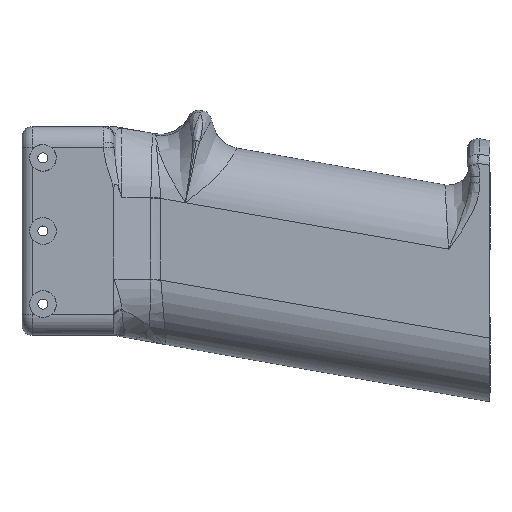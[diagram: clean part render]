
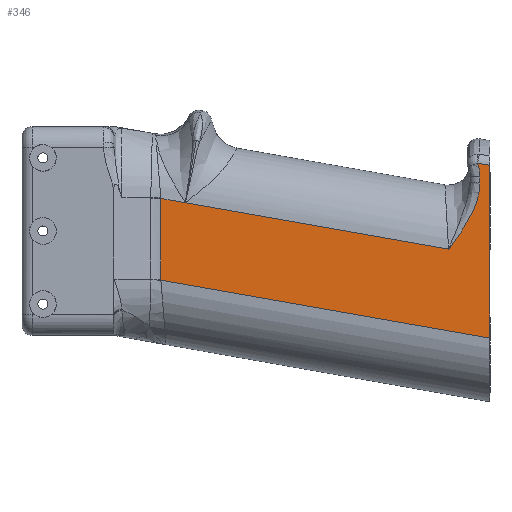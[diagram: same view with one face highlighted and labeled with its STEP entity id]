
A CAD part, left-side view. The second image highlights one B-rep face of the part: STEP entity #346.
In plain terms, the highlighted planar face has unit normal (-1, 0, 0).
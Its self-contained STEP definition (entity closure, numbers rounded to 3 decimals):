
#270 = CARTESIAN_POINT ( 'NONE',  ( 2.5, -96.204, 16.387 ) ) ;
#346 = ADVANCED_FACE ( 'NONE', ( #710 ), #13445, .F. ) ;
#477 = LINE ( 'NONE', #270, #973 ) ;
#658 = LINE ( 'NONE', #7215, #9537 ) ;
#710 = FACE_OUTER_BOUND ( 'NONE', #6651, .T. ) ;
#736 = CARTESIAN_POINT ( 'NONE',  ( 2.5, -97.508, 10.008 ) ) ;
#790 = CARTESIAN_POINT ( 'NONE',  ( 2.5, -91.197, -2.863 ) ) ;
#973 = VECTOR ( 'NONE', #2447, 1000. ) ;
#1314 = VECTOR ( 'NONE', #1765, 1000. ) ;
#1408 = VERTEX_POINT ( 'NONE', #7202 ) ;
#1598 = CARTESIAN_POINT ( 'NONE',  ( 2.5, -97.358, 15.166 ) ) ;
#1765 = DIRECTION ( 'NONE',  ( 0., -0.985, -0.174 ) ) ;
#1837 = CARTESIAN_POINT ( 'NONE',  ( 2.5, -97.089, 7.821 ) ) ;
#1891 = CARTESIAN_POINT ( 'NONE',  ( 2.5, -90.525, -3.757 ) ) ;
#1935 = AXIS2_PLACEMENT_3D ( 'NONE', #3222, #5436, #13278 ) ;
#2315 = ORIENTED_EDGE ( 'NONE', *, *, #8840, .T. ) ;
#2447 = DIRECTION ( 'NONE',  ( 0., 0.985, 0.174 ) ) ;
#2693 = CARTESIAN_POINT ( 'NONE',  ( 2.5, -97.045, 16.238 ) ) ;
#2938 = CARTESIAN_POINT ( 'NONE',  ( 2.5, -96.634, 6.394 ) ) ;
#2992 = CARTESIAN_POINT ( 'NONE',  ( 2.5, -90.076, -4.351 ) ) ;
#3032 = VERTEX_POINT ( 'NONE', #5212 ) ;
#3222 = CARTESIAN_POINT ( 'NONE',  ( 2.5, 0., 0. ) ) ;
#3355 = B_SPLINE_CURVE_WITH_KNOTS ( 'NONE', 3,
 ( #2693, #9394, #1598, #10521, #3806, #11645 ),
 .UNSPECIFIED., .F., .F.,
 ( 4, 2, 4 ),
 ( 0.001, 0.003, 0.004 ),
 .UNSPECIFIED. ) ;
#3390 = CARTESIAN_POINT ( 'NONE',  ( 2.5, -100., 15.717 ) ) ;
#3616 = CARTESIAN_POINT ( 'NONE',  ( 2.5, -97.576, 12.93 ) ) ;
#3806 = CARTESIAN_POINT ( 'NONE',  ( 2.5, -97.576, 13.493 ) ) ;
#4048 = CARTESIAN_POINT ( 'NONE',  ( 2.5, -96.231, 5.351 ) ) ;
#4054 = ORIENTED_EDGE ( 'NONE', *, *, #8875, .T. ) ;
#4249 = LINE ( 'NONE', #7754, #8971 ) ;
#4265 = VERTEX_POINT ( 'NONE', #5051 ) ;
#4573 = LINE ( 'NONE', #7622, #4764 ) ;
#4590 = LINE ( 'NONE', #7664, #10341 ) ;
#4764 = VECTOR ( 'NONE', #13195, 1000. ) ;
#5037 = CARTESIAN_POINT ( 'NONE',  ( 2.5, -102.605, -26.097 ) ) ;
#5051 = CARTESIAN_POINT ( 'NONE',  ( 2.5, -21.231, -11.749 ) ) ;
#5156 = EDGE_CURVE ( 'NONE', #1408, #5998, #4573, .T. ) ;
#5162 = CARTESIAN_POINT ( 'NONE',  ( 2.5, -95.455, 3.667 ) ) ;
#5212 = CARTESIAN_POINT ( 'NONE',  ( 2.5, -97.576, 11.502 ) ) ;
#5325 = CARTESIAN_POINT ( 'NONE',  ( 2.5, -21.231, -11.532 ) ) ;
#5436 = DIRECTION ( 'NONE',  ( 1., 0., 0. ) ) ;
#5453 = VERTEX_POINT ( 'NONE', #9085 ) ;
#5476 = DIRECTION ( 'NONE',  ( 0., 0.985, 0.174 ) ) ;
#5529 = ORIENTED_EDGE ( 'NONE', *, *, #8603, .T. ) ;
#5998 = VERTEX_POINT ( 'NONE', #3390 ) ;
#6101 = VERTEX_POINT ( 'NONE', #12382 ) ;
#6236 = CARTESIAN_POINT ( 'NONE',  ( 2.5, -97.576, 11.502 ) ) ;
#6289 = CARTESIAN_POINT ( 'NONE',  ( 2.5, -93.584, 0.468 ) ) ;
#6455 = CARTESIAN_POINT ( 'NONE',  ( 2.5, -21.233, -11.677 ) ) ;
#6651 = EDGE_LOOP ( 'NONE', ( #7149, #7364, #7571, #7745, #7908, #5529, #13469, #2315, #4054, #9838 ) ) ;
#6999 = B_SPLINE_CURVE_WITH_KNOTS ( 'NONE', 3,
 ( #5325, #13115, #6455, #14256 ),
 .UNSPECIFIED., .F., .F.,
 ( 4, 4 ),
 ( 0., 0. ),
 .UNSPECIFIED. ) ;
#7149 = ORIENTED_EDGE ( 'NONE', *, *, #7722, .T. ) ;
#7202 = CARTESIAN_POINT ( 'NONE',  ( 2.5, -100., -25.638 ) ) ;
#7215 = CARTESIAN_POINT ( 'NONE',  ( 2.5, -97.576, 0. ) ) ;
#7364 = ORIENTED_EDGE ( 'NONE', *, *, #7913, .T. ) ;
#7430 = CARTESIAN_POINT ( 'NONE',  ( 2.5, -91.863, -1.965 ) ) ;
#7571 = ORIENTED_EDGE ( 'NONE', *, *, #8158, .T. ) ;
#7622 = CARTESIAN_POINT ( 'NONE',  ( 2.5, -100., -40.869 ) ) ;
#7664 = CARTESIAN_POINT ( 'NONE',  ( 2.5, -1.972, 11.184 ) ) ;
#7722 = EDGE_CURVE ( 'NONE', #6101, #5453, #4590, .T. ) ;
#7745 = ORIENTED_EDGE ( 'NONE', *, *, #8390, .T. ) ;
#7754 = CARTESIAN_POINT ( 'NONE',  ( 2.5, -1.972, 11.184 ) ) ;
#7908 = ORIENTED_EDGE ( 'NONE', *, *, #5156, .T. ) ;
#7913 = EDGE_CURVE ( 'NONE', #5453, #8761, #10713, .T. ) ;
#8158 = EDGE_CURVE ( 'NONE', #8761, #4265, #6999, .T. ) ;
#8273 = CARTESIAN_POINT ( 'NONE',  ( 2.5, -21.231, -11.532 ) ) ;
#8390 = EDGE_CURVE ( 'NONE', #4265, #1408, #12632, .T. ) ;
#8519 = CARTESIAN_POINT ( 'NONE',  ( 2.5, -97.265, 8.544 ) ) ;
#8573 = CARTESIAN_POINT ( 'NONE',  ( 2.5, -90.973, -3.161 ) ) ;
#8580 = EDGE_CURVE ( 'NONE', #14193, #6101, #4249, .T. ) ;
#8603 = EDGE_CURVE ( 'NONE', #5998, #10148, #477, .T. ) ;
#8753 = EDGE_CURVE ( 'NONE', #10148, #12235, #3355, .T. ) ;
#8761 = VERTEX_POINT ( 'NONE', #8273 ) ;
#8840 = EDGE_CURVE ( 'NONE', #12235, #3032, #658, .T. ) ;
#8875 = EDGE_CURVE ( 'NONE', #3032, #14193, #13808, .T. ) ;
#8971 = VECTOR ( 'NONE', #5476, 1000. ) ;
#9085 = CARTESIAN_POINT ( 'NONE',  ( 2.5, -21.231, 7.788 ) ) ;
#9394 = CARTESIAN_POINT ( 'NONE',  ( 2.5, -97.225, 15.71 ) ) ;
#9401 = DIRECTION ( 'NONE',  ( 0., 0., -1. ) ) ;
#9488 = DIRECTION ( 'NONE',  ( 0., 0., -1. ) ) ;
#9537 = VECTOR ( 'NONE', #9488, 1000. ) ;
#9646 = CARTESIAN_POINT ( 'NONE',  ( 2.5, -96.757, 6.749 ) ) ;
#9703 = CARTESIAN_POINT ( 'NONE',  ( 2.5, -90.3, -4.055 ) ) ;
#9838 = ORIENTED_EDGE ( 'NONE', *, *, #8580, .T. ) ;
#10148 = VERTEX_POINT ( 'NONE', #13692 ) ;
#10341 = VECTOR ( 'NONE', #11061, 1000. ) ;
#10521 = CARTESIAN_POINT ( 'NONE',  ( 2.5, -97.534, 14.053 ) ) ;
#10713 = LINE ( 'NONE', #12860, #11100 ) ;
#10780 = CARTESIAN_POINT ( 'NONE',  ( 2.5, -96.371, 5.695 ) ) ;
#11061 = DIRECTION ( 'NONE',  ( 0., 0.985, 0.174 ) ) ;
#11100 = VECTOR ( 'NONE', #9401, 1000. ) ;
#11645 = CARTESIAN_POINT ( 'NONE',  ( 2.5, -97.576, 12.93 ) ) ;
#11887 = CARTESIAN_POINT ( 'NONE',  ( 2.5, -95.785, 4.33 ) ) ;
#12235 = VERTEX_POINT ( 'NONE', #3616 ) ;
#12382 = CARTESIAN_POINT ( 'NONE',  ( 2.5, -27.091, 6.755 ) ) ;
#12632 = LINE ( 'NONE', #5037, #1314 ) ;
#12860 = CARTESIAN_POINT ( 'NONE',  ( 2.5, -21.231, -11.532 ) ) ;
#13002 = CARTESIAN_POINT ( 'NONE',  ( 2.5, -94.392, 1.717 ) ) ;
#13112 = CARTESIAN_POINT ( 'NONE',  ( 2.5, -90.076, -4.351 ) ) ;
#13115 = CARTESIAN_POINT ( 'NONE',  ( 2.5, -21.233, -11.604 ) ) ;
#13195 = DIRECTION ( 'NONE',  ( 0., 0., 1. ) ) ;
#13278 = DIRECTION ( 'NONE',  ( 0., 0., -1. ) ) ;
#13445 = PLANE ( 'NONE',  #1935 ) ;
#13469 = ORIENTED_EDGE ( 'NONE', *, *, #8753, .T. ) ;
#13692 = CARTESIAN_POINT ( 'NONE',  ( 2.5, -97.045, 16.238 ) ) ;
#13808 = B_SPLINE_CURVE_WITH_KNOTS ( 'NONE', 3,
 ( #6236, #13942, #736, #8519, #1837, #9646, #2938, #10780, #4048, #11887, #5162, #13002, #6289, #14100, #7430, #790, #8573, #1891, #9703, #2992 ),
 .UNSPECIFIED., .F., .F.,
 ( 4, 2, 2, 2, 2, 2, 2, 2, 2, 4 ),
 ( 0., 0.002, 0.004, 0.006, 0.007, 0.009, 0.013, 0.016, 0.017, 0.018 ),
 .UNSPECIFIED. ) ;
#13942 = CARTESIAN_POINT ( 'NONE',  ( 2.5, -97.576, 10.749 ) ) ;
#14100 = CARTESIAN_POINT ( 'NONE',  ( 2.5, -92.301, -1.363 ) ) ;
#14193 = VERTEX_POINT ( 'NONE', #13112 ) ;
#14256 = CARTESIAN_POINT ( 'NONE',  ( 2.5, -21.231, -11.749 ) ) ;
